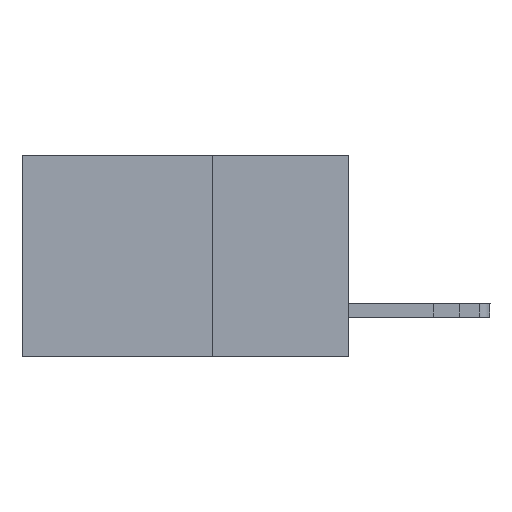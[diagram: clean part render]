
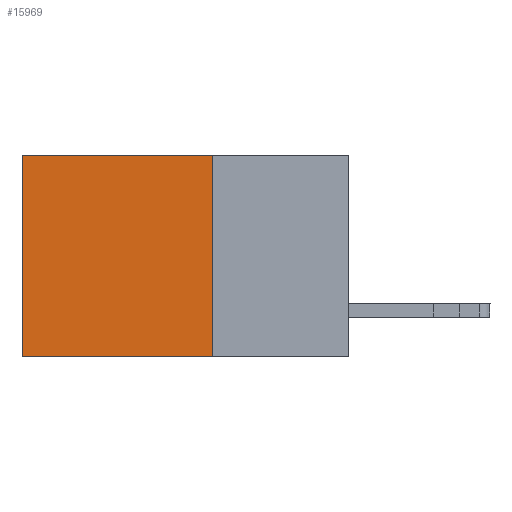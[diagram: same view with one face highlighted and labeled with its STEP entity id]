
A CAD part, left-side view. The second image highlights one B-rep face of the part: STEP entity #15969.
In plain terms, the highlighted planar face has unit normal (-1, 0, 0).
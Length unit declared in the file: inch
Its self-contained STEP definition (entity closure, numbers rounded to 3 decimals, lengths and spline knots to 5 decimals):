
#364 = EDGE_CURVE ( 'NONE', #16496, #5746, #10680, .T. ) ;
#1763 = CARTESIAN_POINT ( 'NONE',  ( 0.2615, 0.25, -0.37 ) ) ;
#2620 = ORIENTED_EDGE ( 'NONE', *, *, #3028, .T. ) ;
#3028 = EDGE_CURVE ( 'NONE', #16496, #5367, #7806, .T. ) ;
#3110 = CARTESIAN_POINT ( 'NONE',  ( 0.2615, 0.6, -0.37 ) ) ;
#3850 = CARTESIAN_POINT ( 'NONE',  ( 0.2615, 0.6, -0.37 ) ) ;
#3887 = DIRECTION ( 'NONE',  ( 0., 1., 0. ) ) ;
#4745 = VECTOR ( 'NONE', #3887, 39.37008 ) ;
#5346 = PLANE ( 'NONE',  #6152 ) ;
#5367 = VERTEX_POINT ( 'NONE', #12276 ) ;
#5694 = DIRECTION ( 'NONE',  ( 0., 0., -1. ) ) ;
#5746 = VERTEX_POINT ( 'NONE', #6707 ) ;
#5879 = CARTESIAN_POINT ( 'NONE',  ( 0.2615, 0.25, -0.37 ) ) ;
#5889 = VECTOR ( 'NONE', #15376, 39.37008 ) ;
#6152 = AXIS2_PLACEMENT_3D ( 'NONE', #1763, #17499, #7129 ) ;
#6707 = CARTESIAN_POINT ( 'NONE',  ( 0.2615, 0.25, -0.37 ) ) ;
#7129 = DIRECTION ( 'NONE',  ( 0., 0., -1. ) ) ;
#7806 = LINE ( 'NONE', #22254, #13570 ) ;
#8102 = VERTEX_POINT ( 'NONE', #3850 ) ;
#8110 = ORIENTED_EDGE ( 'NONE', *, *, #14573, .T. ) ;
#8940 = FACE_OUTER_BOUND ( 'NONE', #16058, .T. ) ;
#9438 = LINE ( 'NONE', #14382, #4745 ) ;
#10023 = LINE ( 'NONE', #3110, #5889 ) ;
#10680 = LINE ( 'NONE', #5879, #19842 ) ;
#12276 = CARTESIAN_POINT ( 'NONE',  ( 0.2615, 0.6, 0. ) ) ;
#13039 = ORIENTED_EDGE ( 'NONE', *, *, #15416, .F. ) ;
#13570 = VECTOR ( 'NONE', #22074, 39.37008 ) ;
#14382 = CARTESIAN_POINT ( 'NONE',  ( 0.2615, 0.25, -0.37 ) ) ;
#14573 = EDGE_CURVE ( 'NONE', #5367, #8102, #10023, .T. ) ;
#15376 = DIRECTION ( 'NONE',  ( 0., 0., -1. ) ) ;
#15416 = EDGE_CURVE ( 'NONE', #5746, #8102, #9438, .T. ) ;
#15969 = ADVANCED_FACE ( 'NONE', ( #8940 ), #5346, .F. ) ;
#16058 = EDGE_LOOP ( 'NONE', ( #8110, #13039, #20115, #2620 ) ) ;
#16496 = VERTEX_POINT ( 'NONE', #22273 ) ;
#17499 = DIRECTION ( 'NONE',  ( 1., 0., 0. ) ) ;
#19842 = VECTOR ( 'NONE', #5694, 39.37008 ) ;
#20115 = ORIENTED_EDGE ( 'NONE', *, *, #364, .F. ) ;
#22074 = DIRECTION ( 'NONE',  ( 0., 1., 0. ) ) ;
#22254 = CARTESIAN_POINT ( 'NONE',  ( 0.2615, 0.25, 0. ) ) ;
#22273 = CARTESIAN_POINT ( 'NONE',  ( 0.2615, 0.25, 0. ) ) ;
